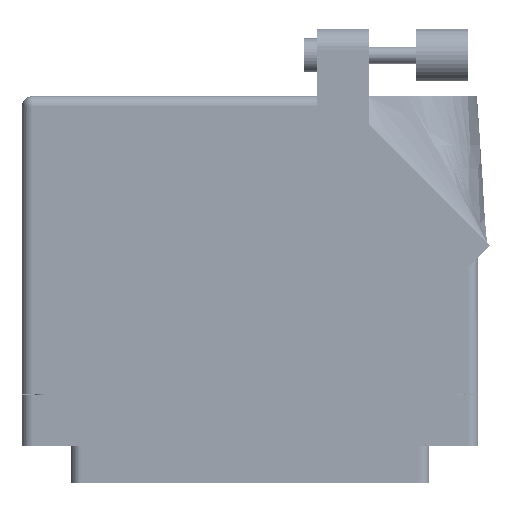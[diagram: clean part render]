
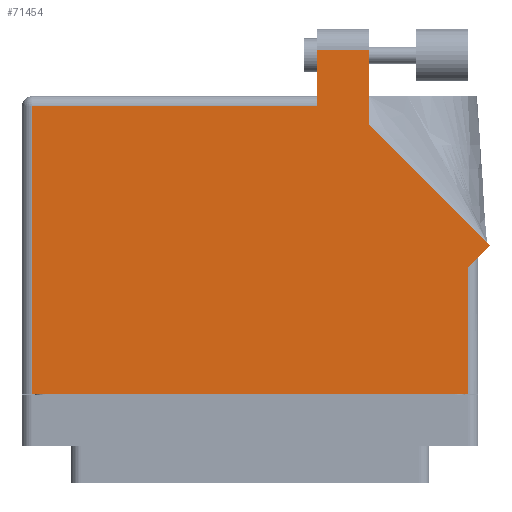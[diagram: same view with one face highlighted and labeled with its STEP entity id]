
A CAD part, front view. The second image highlights one B-rep face of the part: STEP entity #71454.
In plain terms, the highlighted face is planar.
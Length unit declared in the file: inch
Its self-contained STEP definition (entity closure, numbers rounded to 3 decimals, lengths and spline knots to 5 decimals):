
#894 = LINE ( 'NONE', #35397, #66142 ) ;
#1401 = EDGE_CURVE ( 'NONE', #45899, #52662, #47919, .T. ) ;
#2139 = CARTESIAN_POINT ( 'NONE',  ( -1.359, 1.675, 0.617 ) ) ;
#2333 = CARTESIAN_POINT ( 'NONE',  ( -1.297, -0.1, 0.617 ) ) ;
#2586 = EDGE_CURVE ( 'NONE', #50267, #18025, #65853, .T. ) ;
#3604 = VECTOR ( 'NONE', #52853, 39.37008 ) ;
#3808 = CARTESIAN_POINT ( 'NONE',  ( 0.706, 1.95, 0.617 ) ) ;
#4102 = EDGE_CURVE ( 'NONE', #52662, #47822, #894, .T. ) ;
#4527 = CARTESIAN_POINT ( 'NONE',  ( 0.706, 1.50942, 0.617 ) ) ;
#7153 = DIRECTION ( 'NONE',  ( 0., -1., 0. ) ) ;
#8730 = CARTESIAN_POINT ( 'NONE',  ( -1.359, -0.1, 0.617 ) ) ;
#8834 = DIRECTION ( 'NONE',  ( -1., 0., 0. ) ) ;
#10585 = CARTESIAN_POINT ( 'NONE',  ( 0.706, 1.50942, 0.617 ) ) ;
#11706 = EDGE_CURVE ( 'NONE', #18025, #14682, #39660, .T. ) ;
#14527 = CARTESIAN_POINT ( 'NONE',  ( 0.399, 1.95, 0.617 ) ) ;
#14682 = VERTEX_POINT ( 'NONE', #66295 ) ;
#15033 = DIRECTION ( 'NONE',  ( -1., 0., 0. ) ) ;
#15319 = EDGE_CURVE ( 'NONE', #24719, #45899, #39115, .T. ) ;
#18025 = VERTEX_POINT ( 'NONE', #21339 ) ;
#18564 = FACE_OUTER_BOUND ( 'NONE', #18633, .T. ) ;
#18633 = EDGE_LOOP ( 'NONE', ( #60001, #68393, #21577, #20806, #47470, #39898, #41669, #66155, #60820 ) ) ;
#19315 = PLANE ( 'NONE',  #30342 ) ;
#19510 = VECTOR ( 'NONE', #44464, 39.37008 ) ;
#20773 = LINE ( 'NONE', #28863, #43049 ) ;
#20806 = ORIENTED_EDGE ( 'NONE', *, *, #31980, .T. ) ;
#20918 = CARTESIAN_POINT ( 'NONE',  ( -1.297, -0.1, 0.617 ) ) ;
#21339 = CARTESIAN_POINT ( 'NONE',  ( 1.297, 0.653, 0.617 ) ) ;
#21577 = ORIENTED_EDGE ( 'NONE', *, *, #4102, .T. ) ;
#24444 = CARTESIAN_POINT ( 'NONE',  ( 0.399, 1.613, 0.617 ) ) ;
#24719 = VERTEX_POINT ( 'NONE', #10585 ) ;
#25391 = EDGE_CURVE ( 'NONE', #44814, #50267, #55306, .T. ) ;
#25685 = DIRECTION ( 'NONE',  ( 1., 0., 0. ) ) ;
#26481 = VECTOR ( 'NONE', #15033, 39.37008 ) ;
#28863 = CARTESIAN_POINT ( 'NONE',  ( 1.42971, 0.78571, 0.617 ) ) ;
#29046 = CARTESIAN_POINT ( 'NONE',  ( 0.399, 1.95, 0.617 ) ) ;
#29051 = CARTESIAN_POINT ( 'NONE',  ( -1.297, 1.613, 0.617 ) ) ;
#30234 = VECTOR ( 'NONE', #25685, 39.37008 ) ;
#30342 = AXIS2_PLACEMENT_3D ( 'NONE', #2139, #54054, #8834 ) ;
#31980 = EDGE_CURVE ( 'NONE', #47822, #49072, #64353, .T. ) ;
#35088 = DIRECTION ( 'NONE',  ( -0.707, 0.707, 0. ) ) ;
#35397 = CARTESIAN_POINT ( 'NONE',  ( 0.399, 1.675, 0.617 ) ) ;
#39115 = LINE ( 'NONE', #4527, #19510 ) ;
#39660 = LINE ( 'NONE', #70162, #51284 ) ;
#39898 = ORIENTED_EDGE ( 'NONE', *, *, #25391, .T. ) ;
#41669 = ORIENTED_EDGE ( 'NONE', *, *, #2586, .T. ) ;
#42475 = DIRECTION ( 'NONE',  ( 0., -1., 0. ) ) ;
#42621 = DIRECTION ( 'NONE',  ( 0., 1., 0. ) ) ;
#43049 = VECTOR ( 'NONE', #35088, 39.37008 ) ;
#44464 = DIRECTION ( 'NONE',  ( 0., 1., 0. ) ) ;
#44600 = LINE ( 'NONE', #2333, #69584 ) ;
#44814 = VERTEX_POINT ( 'NONE', #20918 ) ;
#45899 = VERTEX_POINT ( 'NONE', #3808 ) ;
#47470 = ORIENTED_EDGE ( 'NONE', *, *, #61932, .T. ) ;
#47822 = VERTEX_POINT ( 'NONE', #24444 ) ;
#47919 = LINE ( 'NONE', #14527, #26481 ) ;
#49072 = VERTEX_POINT ( 'NONE', #29051 ) ;
#50267 = VERTEX_POINT ( 'NONE', #54924 ) ;
#50643 = VECTOR ( 'NONE', #42621, 39.37008 ) ;
#51284 = VECTOR ( 'NONE', #53470, 39.37008 ) ;
#52194 = CARTESIAN_POINT ( 'NONE',  ( 1.297, 0.715, 0.617 ) ) ;
#52662 = VERTEX_POINT ( 'NONE', #29046 ) ;
#52853 = DIRECTION ( 'NONE',  ( -1., 0., 0. ) ) ;
#53470 = DIRECTION ( 'NONE',  ( 0.707, 0.707, 0. ) ) ;
#54054 = DIRECTION ( 'NONE',  ( 0., 0., -1. ) ) ;
#54924 = CARTESIAN_POINT ( 'NONE',  ( 1.297, -0.1, 0.617 ) ) ;
#55306 = LINE ( 'NONE', #8730, #30234 ) ;
#60001 = ORIENTED_EDGE ( 'NONE', *, *, #15319, .T. ) ;
#60820 = ORIENTED_EDGE ( 'NONE', *, *, #73903, .T. ) ;
#61932 = EDGE_CURVE ( 'NONE', #49072, #44814, #44600, .T. ) ;
#64353 = LINE ( 'NONE', #70579, #3604 ) ;
#65853 = LINE ( 'NONE', #52194, #50643 ) ;
#66142 = VECTOR ( 'NONE', #7153, 39.37008 ) ;
#66155 = ORIENTED_EDGE ( 'NONE', *, *, #11706, .T. ) ;
#66295 = CARTESIAN_POINT ( 'NONE',  ( 1.42971, 0.78571, 0.617 ) ) ;
#68393 = ORIENTED_EDGE ( 'NONE', *, *, #1401, .T. ) ;
#69584 = VECTOR ( 'NONE', #42475, 39.37008 ) ;
#70162 = CARTESIAN_POINT ( 'NONE',  ( 1.359, 0.715, 0.617 ) ) ;
#70579 = CARTESIAN_POINT ( 'NONE',  ( -1.359, 1.613, 0.617 ) ) ;
#71454 = ADVANCED_FACE ( 'NONE', ( #18564 ), #19315, .F. ) ;
#73903 = EDGE_CURVE ( 'NONE', #14682, #24719, #20773, .T. ) ;
